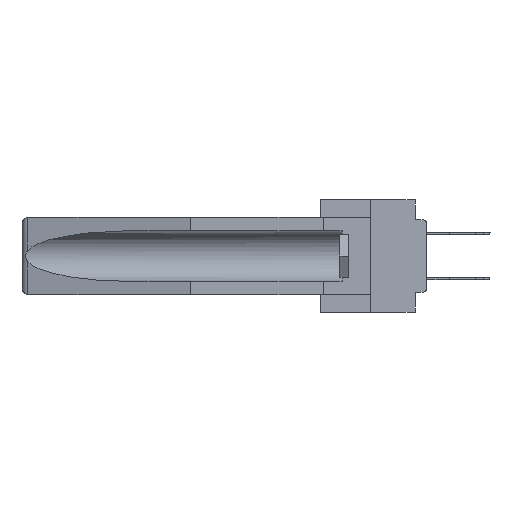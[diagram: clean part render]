
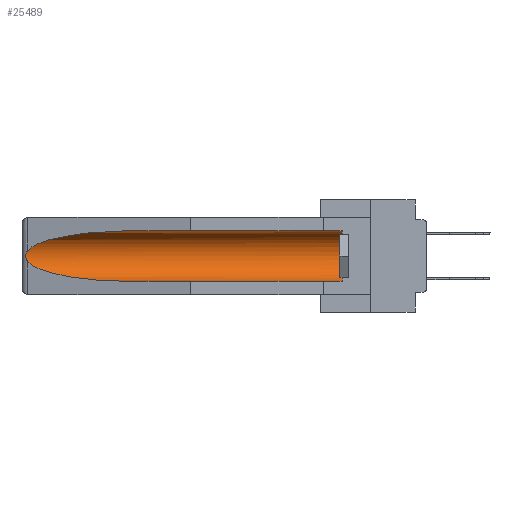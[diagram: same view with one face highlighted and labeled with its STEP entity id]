
A CAD part, left-side view. The second image highlights one B-rep face of the part: STEP entity #25489.
In plain terms, the highlighted cylindrical face has radius 2.857 mm (diameter 5.715 mm), a partial arc.
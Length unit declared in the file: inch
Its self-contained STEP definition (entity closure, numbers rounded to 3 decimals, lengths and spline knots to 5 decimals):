
#32 = B_SPLINE_CURVE_WITH_KNOTS ( 'NONE', 3,
 ( #20598, #25463, #5081, #13698, #18661, #7343, #16099, #27891, #22908, #9610 ),
 .UNSPECIFIED., .F., .F.,
 ( 4, 2, 2, 2, 4 ),
 ( 0., 0.00029, 0.00058, 0.00087, 0.00117 ),
 .UNSPECIFIED. ) ;
#1245 = AXIS2_PLACEMENT_3D ( 'NONE', #6170, #8890, #2108 ) ;
#2108 = DIRECTION ( 'NONE',  ( 0., 0., 1. ) ) ;
#2455 = DIRECTION ( 'NONE',  ( 0., 0., 1. ) ) ;
#2911 = VERTEX_POINT ( 'NONE', #25116 ) ;
#3064 =( BOUNDED_CURVE ( )  B_SPLINE_CURVE ( 3, ( #6865, #16366, #20712, #24980 ),
 .UNSPECIFIED., .F., .F. ) 
 B_SPLINE_CURVE_WITH_KNOTS ( ( 4, 4 ),
 ( 4.71239, 6.08839 ),
 .UNSPECIFIED. ) 
 CURVE ( )  GEOMETRIC_REPRESENTATION_ITEM ( )  RATIONAL_B_SPLINE_CURVE ( ( 1., 0.848, 0.848, 1. ) ) 
 REPRESENTATION_ITEM ( '' )  );
#4331 = ORIENTED_EDGE ( 'NONE', *, *, #11894, .F. ) ;
#4657 = VECTOR ( 'NONE', #26047, 39.37008 ) ;
#5081 = CARTESIAN_POINT ( 'NONE',  ( 0.26654, 1.53092, -0.15636 ) ) ;
#6170 = CARTESIAN_POINT ( 'NONE',  ( 0.155, 0.126, -0.1715 ) ) ;
#6519 = VERTEX_POINT ( 'NONE', #21490 ) ;
#6865 = CARTESIAN_POINT ( 'NONE',  ( 0.155, 1.07973, -0.059 ) ) ;
#7343 = CARTESIAN_POINT ( 'NONE',  ( 0.2675, 1.53308, -0.17534 ) ) ;
#8396 = CARTESIAN_POINT ( 'NONE',  ( 0.155, 1.07973, -0.059 ) ) ;
#8488 = ORIENTED_EDGE ( 'NONE', *, *, #13852, .T. ) ;
#8573 = EDGE_CURVE ( 'NONE', #6519, #15777, #15671, .T. ) ;
#8890 = DIRECTION ( 'NONE',  ( 0., -1., 0. ) ) ;
#9113 = EDGE_CURVE ( 'NONE', #26639, #25337, #3064, .T. ) ;
#9610 = CARTESIAN_POINT ( 'NONE',  ( 0.26537, 1.52718, -0.19328 ) ) ;
#10599 = VERTEX_POINT ( 'NONE', #24804 ) ;
#11635 = CARTESIAN_POINT ( 'NONE',  ( 0.26537, 1.52718, -0.19328 ) ) ;
#11894 = EDGE_CURVE ( 'NONE', #6519, #2911, #14421, .T. ) ;
#11939 = FACE_OUTER_BOUND ( 'NONE', #13921, .T. ) ;
#13698 = CARTESIAN_POINT ( 'NONE',  ( 0.2673, 1.5327, -0.16383 ) ) ;
#13852 = EDGE_CURVE ( 'NONE', #10599, #2911, #28896, .T. ) ;
#13912 = CARTESIAN_POINT ( 'NONE',  ( 0.25451, 1.48313, -0.24835 ) ) ;
#13921 = EDGE_LOOP ( 'NONE', ( #25708, #24013, #8488, #4331, #20997, #29406 ) ) ;
#14335 = LINE ( 'NONE', #18393, #19070 ) ;
#14421 = LINE ( 'NONE', #16827, #4657 ) ;
#15671 = CIRCLE ( 'NONE', #1245, 0.1125 ) ;
#15777 = VERTEX_POINT ( 'NONE', #16594 ) ;
#16099 = CARTESIAN_POINT ( 'NONE',  ( 0.2673, 1.53269, -0.17917 ) ) ;
#16366 = CARTESIAN_POINT ( 'NONE',  ( 0.21114, 1.30732, -0.059 ) ) ;
#16594 = CARTESIAN_POINT ( 'NONE',  ( 0.155, 0.126, -0.059 ) ) ;
#16827 = CARTESIAN_POINT ( 'NONE',  ( 0.155, -0.30754, -0.284 ) ) ;
#18393 = CARTESIAN_POINT ( 'NONE',  ( 0.155, -0.30754, -0.059 ) ) ;
#18661 = CARTESIAN_POINT ( 'NONE',  ( 0.2675, 1.53308, -0.16763 ) ) ;
#19070 = VECTOR ( 'NONE', #23239, 39.37008 ) ;
#20216 = CARTESIAN_POINT ( 'NONE',  ( 0.21114, 1.30732, -0.284 ) ) ;
#20598 = CARTESIAN_POINT ( 'NONE',  ( 0.26537, 1.52718, -0.14972 ) ) ;
#20657 = CARTESIAN_POINT ( 'NONE',  ( 0.155, 1.07973, -0.284 ) ) ;
#20712 = CARTESIAN_POINT ( 'NONE',  ( 0.25451, 1.48313, -0.09465 ) ) ;
#20997 = ORIENTED_EDGE ( 'NONE', *, *, #8573, .T. ) ;
#21108 = DIRECTION ( 'NONE',  ( 0., 1., 0. ) ) ;
#21490 = CARTESIAN_POINT ( 'NONE',  ( 0.155, 0.126, -0.284 ) ) ;
#22423 = CARTESIAN_POINT ( 'NONE',  ( 0.26537, 1.52718, -0.14972 ) ) ;
#22908 = CARTESIAN_POINT ( 'NONE',  ( 0.26597, 1.5296, -0.19026 ) ) ;
#23108 = CARTESIAN_POINT ( 'NONE',  ( 0.155, -0.30754, -0.1715 ) ) ;
#23239 = DIRECTION ( 'NONE',  ( 0., 1., 0. ) ) ;
#23265 = CYLINDRICAL_SURFACE ( 'NONE', #23850, 0.1125 ) ;
#23850 = AXIS2_PLACEMENT_3D ( 'NONE', #23108, #21108, #2455 ) ;
#24013 = ORIENTED_EDGE ( 'NONE', *, *, #27611, .T. ) ;
#24804 = CARTESIAN_POINT ( 'NONE',  ( 0.26537, 1.52718, -0.19328 ) ) ;
#24980 = CARTESIAN_POINT ( 'NONE',  ( 0.26537, 1.52718, -0.14972 ) ) ;
#25116 = CARTESIAN_POINT ( 'NONE',  ( 0.155, 1.07973, -0.284 ) ) ;
#25337 = VERTEX_POINT ( 'NONE', #22423 ) ;
#25463 = CARTESIAN_POINT ( 'NONE',  ( 0.26597, 1.52961, -0.15275 ) ) ;
#25489 = ADVANCED_FACE ( 'NONE', ( #11939 ), #23265, .F. ) ;
#25708 = ORIENTED_EDGE ( 'NONE', *, *, #9113, .T. ) ;
#26047 = DIRECTION ( 'NONE',  ( 0., 1., 0. ) ) ;
#26639 = VERTEX_POINT ( 'NONE', #8396 ) ;
#27157 = EDGE_CURVE ( 'NONE', #15777, #26639, #14335, .T. ) ;
#27611 = EDGE_CURVE ( 'NONE', #25337, #10599, #32, .T. ) ;
#27891 = CARTESIAN_POINT ( 'NONE',  ( 0.26655, 1.53094, -0.18657 ) ) ;
#28896 =( BOUNDED_CURVE ( )  B_SPLINE_CURVE ( 3, ( #11635, #13912, #20216, #20657 ),
 .UNSPECIFIED., .F., .T. ) 
 B_SPLINE_CURVE_WITH_KNOTS ( ( 4, 4 ),
 ( 0.1948, 1.5708 ),
 .UNSPECIFIED. ) 
 CURVE ( )  GEOMETRIC_REPRESENTATION_ITEM ( )  RATIONAL_B_SPLINE_CURVE ( ( 1., 0.848, 0.848, 1. ) ) 
 REPRESENTATION_ITEM ( '' )  );
#29406 = ORIENTED_EDGE ( 'NONE', *, *, #27157, .T. ) ;
